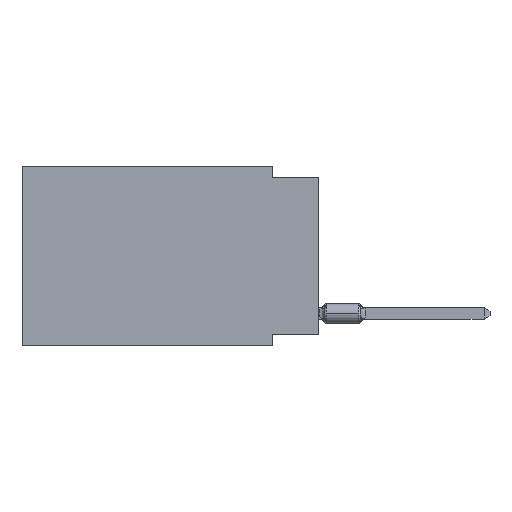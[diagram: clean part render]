
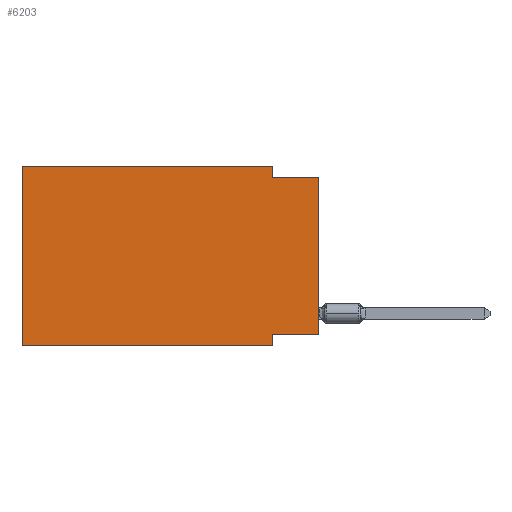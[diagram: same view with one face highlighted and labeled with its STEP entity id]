
A CAD part, left-side view. The second image highlights one B-rep face of the part: STEP entity #6203.
In plain terms, the highlighted planar face has unit normal (-1, 0, 0).
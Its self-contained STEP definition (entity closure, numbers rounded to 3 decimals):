
#347 = DIRECTION ( 'NONE',  ( 0., 0., -1. ) ) ;
#506 = EDGE_CURVE ( 'NONE', #7564, #12005, #11271, .T. ) ;
#833 = DIRECTION ( 'NONE',  ( 0., 0., -1. ) ) ;
#959 = VECTOR ( 'NONE', #5507, 1000. ) ;
#985 = CARTESIAN_POINT ( 'NONE',  ( 0., 16.383, 0. ) ) ;
#1099 = CARTESIAN_POINT ( 'NONE',  ( 0., 0., -0.635 ) ) ;
#1404 = VERTEX_POINT ( 'NONE', #9860 ) ;
#2042 = CARTESIAN_POINT ( 'NONE',  ( 0., 2.54, 0. ) ) ;
#2367 = PLANE ( 'NONE',  #11358 ) ;
#2601 = ORIENTED_EDGE ( 'NONE', *, *, #8259, .F. ) ;
#3683 = EDGE_LOOP ( 'NONE', ( #7642, #9957, #12943, #2601, #15438, #12354, #12962, #15637 ) ) ;
#3701 = VERTEX_POINT ( 'NONE', #1099 ) ;
#4114 = LINE ( 'NONE', #11904, #7117 ) ;
#5109 = CARTESIAN_POINT ( 'NONE',  ( 0., 0., 0. ) ) ;
#5507 = DIRECTION ( 'NONE',  ( 0., 0., 1. ) ) ;
#6041 = CARTESIAN_POINT ( 'NONE',  ( 0., 16.383, -9.906 ) ) ;
#6099 = VERTEX_POINT ( 'NONE', #6041 ) ;
#6203 = ADVANCED_FACE ( 'NONE', ( #6217 ), #2367, .F. ) ;
#6217 = FACE_OUTER_BOUND ( 'NONE', #3683, .T. ) ;
#6701 = DIRECTION ( 'NONE',  ( 0., -1., 0. ) ) ;
#6729 = LINE ( 'NONE', #5109, #959 ) ;
#6946 = DIRECTION ( 'NONE',  ( 0., -1., 0. ) ) ;
#7117 = VECTOR ( 'NONE', #6946, 1000. ) ;
#7302 = EDGE_CURVE ( 'NONE', #11897, #3701, #14130, .T. ) ;
#7564 = VERTEX_POINT ( 'NONE', #10003 ) ;
#7642 = ORIENTED_EDGE ( 'NONE', *, *, #9039, .T. ) ;
#7674 = EDGE_CURVE ( 'NONE', #14762, #11897, #12118, .T. ) ;
#7831 = DIRECTION ( 'NONE',  ( 1., 0., 0. ) ) ;
#7999 = VECTOR ( 'NONE', #13931, 1000. ) ;
#8259 = EDGE_CURVE ( 'NONE', #1404, #14762, #15014, .T. ) ;
#8482 = LINE ( 'NONE', #13698, #9183 ) ;
#8580 = DIRECTION ( 'NONE',  ( 0., -1., 0. ) ) ;
#9039 = EDGE_CURVE ( 'NONE', #7564, #3701, #6729, .T. ) ;
#9183 = VECTOR ( 'NONE', #16443, 1000. ) ;
#9817 = VECTOR ( 'NONE', #833, 1000. ) ;
#9860 = CARTESIAN_POINT ( 'NONE',  ( 0., 16.383, 0. ) ) ;
#9957 = ORIENTED_EDGE ( 'NONE', *, *, #7302, .F. ) ;
#9968 = LINE ( 'NONE', #15204, #9817 ) ;
#10003 = CARTESIAN_POINT ( 'NONE',  ( 0., 0., -9.271 ) ) ;
#10077 = CARTESIAN_POINT ( 'NONE',  ( 0., 0., -9.271 ) ) ;
#10177 = VECTOR ( 'NONE', #347, 1000. ) ;
#10470 = EDGE_CURVE ( 'NONE', #6099, #1404, #8482, .T. ) ;
#11271 = LINE ( 'NONE', #10077, #7999 ) ;
#11347 = DIRECTION ( 'NONE',  ( 0., 0., -1. ) ) ;
#11358 = AXIS2_PLACEMENT_3D ( 'NONE', #15295, #7831, #11347 ) ;
#11470 = EDGE_CURVE ( 'NONE', #12005, #15710, #9968, .T. ) ;
#11625 = CARTESIAN_POINT ( 'NONE',  ( 0., 2.54, -0.635 ) ) ;
#11897 = VERTEX_POINT ( 'NONE', #11625 ) ;
#11904 = CARTESIAN_POINT ( 'NONE',  ( 0., 16.383, -9.906 ) ) ;
#12005 = VERTEX_POINT ( 'NONE', #13159 ) ;
#12118 = LINE ( 'NONE', #13738, #10177 ) ;
#12354 = ORIENTED_EDGE ( 'NONE', *, *, #15416, .T. ) ;
#12826 = CARTESIAN_POINT ( 'NONE',  ( 0., 0., -0.635 ) ) ;
#12943 = ORIENTED_EDGE ( 'NONE', *, *, #7674, .F. ) ;
#12962 = ORIENTED_EDGE ( 'NONE', *, *, #11470, .F. ) ;
#13159 = CARTESIAN_POINT ( 'NONE',  ( 0., 2.54, -9.271 ) ) ;
#13698 = CARTESIAN_POINT ( 'NONE',  ( 0., 16.383, 0. ) ) ;
#13738 = CARTESIAN_POINT ( 'NONE',  ( 0., 2.54, 0. ) ) ;
#13850 = VECTOR ( 'NONE', #6701, 1000. ) ;
#13931 = DIRECTION ( 'NONE',  ( 0., 1., 0. ) ) ;
#14130 = LINE ( 'NONE', #12826, #13850 ) ;
#14283 = CARTESIAN_POINT ( 'NONE',  ( 0., 2.54, -9.906 ) ) ;
#14762 = VERTEX_POINT ( 'NONE', #2042 ) ;
#15014 = LINE ( 'NONE', #985, #15687 ) ;
#15204 = CARTESIAN_POINT ( 'NONE',  ( 0., 2.54, -9.906 ) ) ;
#15295 = CARTESIAN_POINT ( 'NONE',  ( 0., 16.383, 0. ) ) ;
#15416 = EDGE_CURVE ( 'NONE', #6099, #15710, #4114, .T. ) ;
#15438 = ORIENTED_EDGE ( 'NONE', *, *, #10470, .F. ) ;
#15637 = ORIENTED_EDGE ( 'NONE', *, *, #506, .F. ) ;
#15687 = VECTOR ( 'NONE', #8580, 1000. ) ;
#15710 = VERTEX_POINT ( 'NONE', #14283 ) ;
#16443 = DIRECTION ( 'NONE',  ( 0., 0., 1. ) ) ;
